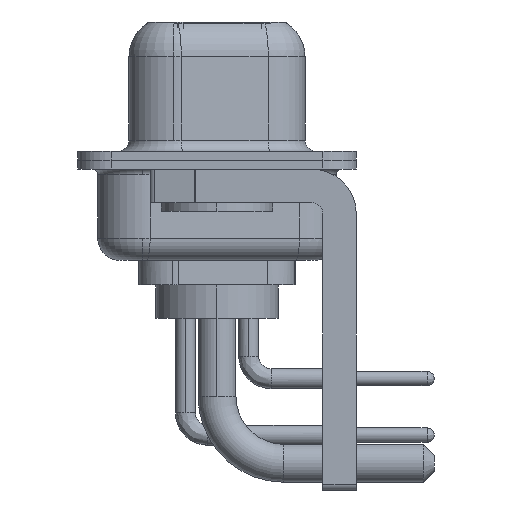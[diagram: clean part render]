
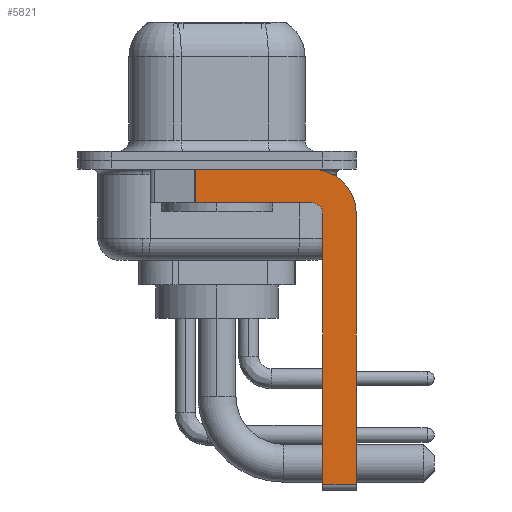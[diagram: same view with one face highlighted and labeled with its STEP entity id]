
A CAD part, left-side view. The second image highlights one B-rep face of the part: STEP entity #5821.
In plain terms, the highlighted planar face has unit normal (-1, 0, 0).
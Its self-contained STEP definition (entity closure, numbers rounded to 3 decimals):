
#70 = CARTESIAN_POINT ( 'NONE',  ( -2.9, -4.25, -1.9 ) ) ;
#128 = EDGE_CURVE ( 'NONE', #16095, #6991, #20885, .T. ) ;
#215 = LINE ( 'NONE', #5535, #2099 ) ;
#313 = ORIENTED_EDGE ( 'NONE', *, *, #12330, .F. ) ;
#447 = VERTEX_POINT ( 'NONE', #9563 ) ;
#793 = DIRECTION ( 'NONE',  ( 0., 0., 1. ) ) ;
#803 = CARTESIAN_POINT ( 'NONE',  ( -2.9, -6.25, -2.4 ) ) ;
#915 = CARTESIAN_POINT ( 'NONE',  ( -2.9, -4.25, -2.4 ) ) ;
#932 = CARTESIAN_POINT ( 'NONE',  ( -2.9, -4.75, -2.4 ) ) ;
#1701 = VERTEX_POINT ( 'NONE', #6593 ) ;
#1881 = DIRECTION ( 'NONE',  ( 0., 0., -1. ) ) ;
#2099 = VECTOR ( 'NONE', #18918, 1000. ) ;
#2185 = ORIENTED_EDGE ( 'NONE', *, *, #19155, .F. ) ;
#2402 = ORIENTED_EDGE ( 'NONE', *, *, #4464, .T. ) ;
#2429 = CARTESIAN_POINT ( 'NONE',  ( -2.9, -6.25, -14.55 ) ) ;
#3237 = DIRECTION ( 'NONE',  ( 0., 0., -1. ) ) ;
#3349 = PLANE ( 'NONE',  #18615 ) ;
#3798 = EDGE_CURVE ( 'NONE', #447, #22299, #9562, .T. ) ;
#3865 = VECTOR ( 'NONE', #4825, 1000. ) ;
#3971 = ORIENTED_EDGE ( 'NONE', *, *, #5396, .F. ) ;
#3992 = CARTESIAN_POINT ( 'NONE',  ( -2.9, 0.978, -0.4 ) ) ;
#4464 = EDGE_CURVE ( 'NONE', #16095, #22299, #7217, .T. ) ;
#4631 = VECTOR ( 'NONE', #9213, 1000. ) ;
#4720 = CARTESIAN_POINT ( 'NONE',  ( -2.9, -4.25, -2.4 ) ) ;
#4825 = DIRECTION ( 'NONE',  ( 0., 0., -1. ) ) ;
#5396 = EDGE_CURVE ( 'NONE', #17552, #1701, #7049, .T. ) ;
#5535 = CARTESIAN_POINT ( 'NONE',  ( -2.9, -4.25, -1.9 ) ) ;
#5674 = ORIENTED_EDGE ( 'NONE', *, *, #20703, .F. ) ;
#5821 = ADVANCED_FACE ( 'NONE', ( #18873 ), #3349, .F. ) ;
#6593 = CARTESIAN_POINT ( 'NONE',  ( -2.9, -4.25, -0.4 ) ) ;
#6804 = VECTOR ( 'NONE', #19265, 1000. ) ;
#6991 = VERTEX_POINT ( 'NONE', #932 ) ;
#7049 = LINE ( 'NONE', #17858, #4631 ) ;
#7214 = AXIS2_PLACEMENT_3D ( 'NONE', #915, #13000, #793 ) ;
#7217 = LINE ( 'NONE', #17793, #14144 ) ;
#7450 = CARTESIAN_POINT ( 'NONE',  ( -2.9, -4.75, -14.55 ) ) ;
#7627 = DIRECTION ( 'NONE',  ( 0., 0., -1. ) ) ;
#9213 = DIRECTION ( 'NONE',  ( 0., -1., 0. ) ) ;
#9562 = LINE ( 'NONE', #803, #11541 ) ;
#9563 = CARTESIAN_POINT ( 'NONE',  ( -2.9, -6.25, -2.4 ) ) ;
#10152 = CIRCLE ( 'NONE', #7214, 0.5 ) ;
#10631 = CARTESIAN_POINT ( 'NONE',  ( -2.9, -4.25, -2.4 ) ) ;
#11541 = VECTOR ( 'NONE', #7627, 1000. ) ;
#11761 = CARTESIAN_POINT ( 'NONE',  ( -2.9, 0.978, -1.9 ) ) ;
#12330 = EDGE_CURVE ( 'NONE', #1701, #447, #20278, .T. ) ;
#13000 = DIRECTION ( 'NONE',  ( -1., 0., 0. ) ) ;
#13291 = EDGE_LOOP ( 'NONE', ( #3971, #15452, #5674, #2185, #17265, #2402, #15010, #313 ) ) ;
#14144 = VECTOR ( 'NONE', #16183, 1000. ) ;
#14950 = CARTESIAN_POINT ( 'NONE',  ( -2.9, 0.978, -1.9 ) ) ;
#15010 = ORIENTED_EDGE ( 'NONE', *, *, #3798, .F. ) ;
#15452 = ORIENTED_EDGE ( 'NONE', *, *, #18435, .T. ) ;
#16095 = VERTEX_POINT ( 'NONE', #7450 ) ;
#16183 = DIRECTION ( 'NONE',  ( 0., -1., 0. ) ) ;
#16761 = VERTEX_POINT ( 'NONE', #11761 ) ;
#17155 = DIRECTION ( 'NONE',  ( 1., 0., 0. ) ) ;
#17205 = CARTESIAN_POINT ( 'NONE',  ( -2.9, -4.75, -14.8 ) ) ;
#17265 = ORIENTED_EDGE ( 'NONE', *, *, #128, .F. ) ;
#17552 = VERTEX_POINT ( 'NONE', #3992 ) ;
#17667 = DIRECTION ( 'NONE',  ( 1., 0., 0. ) ) ;
#17793 = CARTESIAN_POINT ( 'NONE',  ( -2.9, -4.25, -14.55 ) ) ;
#17858 = CARTESIAN_POINT ( 'NONE',  ( -2.9, 3., -0.4 ) ) ;
#18435 = EDGE_CURVE ( 'NONE', #17552, #16761, #20589, .T. ) ;
#18615 = AXIS2_PLACEMENT_3D ( 'NONE', #4720, #17155, #3237 ) ;
#18873 = FACE_OUTER_BOUND ( 'NONE', #13291, .T. ) ;
#18918 = DIRECTION ( 'NONE',  ( 0., 1., 0. ) ) ;
#19155 = EDGE_CURVE ( 'NONE', #6991, #21205, #10152, .T. ) ;
#19265 = DIRECTION ( 'NONE',  ( 0., 0., 1. ) ) ;
#20278 = CIRCLE ( 'NONE', #21759, 2. ) ;
#20589 = LINE ( 'NONE', #14950, #3865 ) ;
#20703 = EDGE_CURVE ( 'NONE', #21205, #16761, #215, .T. ) ;
#20885 = LINE ( 'NONE', #17205, #6804 ) ;
#21205 = VERTEX_POINT ( 'NONE', #70 ) ;
#21759 = AXIS2_PLACEMENT_3D ( 'NONE', #10631, #17667, #1881 ) ;
#22299 = VERTEX_POINT ( 'NONE', #2429 ) ;
